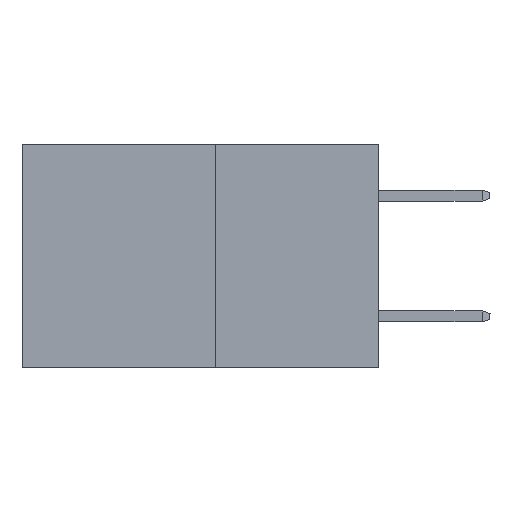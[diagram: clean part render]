
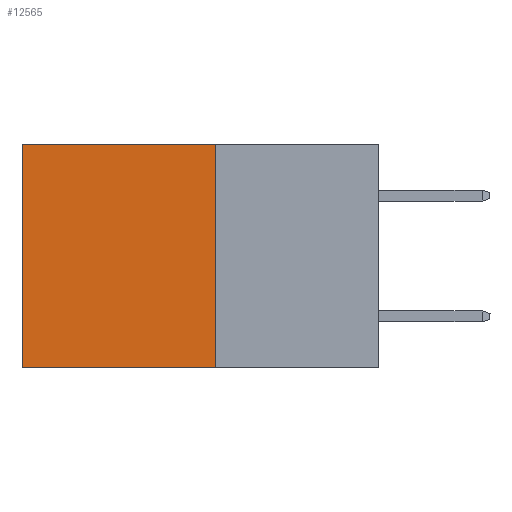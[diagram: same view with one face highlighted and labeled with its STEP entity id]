
A CAD part, left-side view. The second image highlights one B-rep face of the part: STEP entity #12565.
In plain terms, the highlighted planar face has unit normal (-1, 0, 0).
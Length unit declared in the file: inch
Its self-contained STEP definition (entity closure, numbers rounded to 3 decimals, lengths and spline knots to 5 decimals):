
#1158 = CARTESIAN_POINT ( 'NONE',  ( 0.277, 0.27, -0.37 ) ) ;
#2426 = FACE_OUTER_BOUND ( 'NONE', #28629, .T. ) ;
#2497 = VERTEX_POINT ( 'NONE', #19332 ) ;
#4834 = VERTEX_POINT ( 'NONE', #1158 ) ;
#5631 = DIRECTION ( 'NONE',  ( 0., 0., -1. ) ) ;
#5793 = LINE ( 'NONE', #33766, #19429 ) ;
#6070 = VERTEX_POINT ( 'NONE', #28109 ) ;
#7287 = LINE ( 'NONE', #15942, #13672 ) ;
#8657 = VECTOR ( 'NONE', #5631, 39.37008 ) ;
#9258 = EDGE_CURVE ( 'NONE', #33469, #6070, #7287, .T. ) ;
#10693 = DIRECTION ( 'NONE',  ( 0., 0., -1. ) ) ;
#12565 = ADVANCED_FACE ( 'NONE', ( #2426 ), #29597, .F. ) ;
#13358 = ORIENTED_EDGE ( 'NONE', *, *, #24227, .T. ) ;
#13672 = VECTOR ( 'NONE', #29340, 39.37008 ) ;
#13729 = CARTESIAN_POINT ( 'NONE',  ( 0.277, 0.59, -0.37 ) ) ;
#14772 = CARTESIAN_POINT ( 'NONE',  ( 0.277, 0.27, -0.37 ) ) ;
#15942 = CARTESIAN_POINT ( 'NONE',  ( 0.277, 0.27, 0. ) ) ;
#16233 = DIRECTION ( 'NONE',  ( 1., 0., 0. ) ) ;
#17201 = EDGE_CURVE ( 'NONE', #33469, #4834, #33158, .T. ) ;
#19332 = CARTESIAN_POINT ( 'NONE',  ( 0.277, 0.59, -0.37 ) ) ;
#19429 = VECTOR ( 'NONE', #23321, 39.37008 ) ;
#19759 = ORIENTED_EDGE ( 'NONE', *, *, #28875, .F. ) ;
#22918 = DIRECTION ( 'NONE',  ( 0., 0., -1. ) ) ;
#23321 = DIRECTION ( 'NONE',  ( 0., 1., 0. ) ) ;
#24227 = EDGE_CURVE ( 'NONE', #6070, #2497, #30148, .T. ) ;
#25127 = ORIENTED_EDGE ( 'NONE', *, *, #17201, .F. ) ;
#25727 = CARTESIAN_POINT ( 'NONE',  ( 0.277, 0.27, 0. ) ) ;
#26086 = VECTOR ( 'NONE', #22918, 39.37008 ) ;
#28109 = CARTESIAN_POINT ( 'NONE',  ( 0.277, 0.59, 0. ) ) ;
#28629 = EDGE_LOOP ( 'NONE', ( #13358, #19759, #25127, #29552 ) ) ;
#28875 = EDGE_CURVE ( 'NONE', #4834, #2497, #5793, .T. ) ;
#29340 = DIRECTION ( 'NONE',  ( 0., 1., 0. ) ) ;
#29552 = ORIENTED_EDGE ( 'NONE', *, *, #9258, .T. ) ;
#29597 = PLANE ( 'NONE',  #33632 ) ;
#30148 = LINE ( 'NONE', #13729, #8657 ) ;
#32266 = CARTESIAN_POINT ( 'NONE',  ( 0.277, 0.27, -0.37 ) ) ;
#33158 = LINE ( 'NONE', #14772, #26086 ) ;
#33469 = VERTEX_POINT ( 'NONE', #25727 ) ;
#33632 = AXIS2_PLACEMENT_3D ( 'NONE', #32266, #16233, #10693 ) ;
#33766 = CARTESIAN_POINT ( 'NONE',  ( 0.277, 0.27, -0.37 ) ) ;
